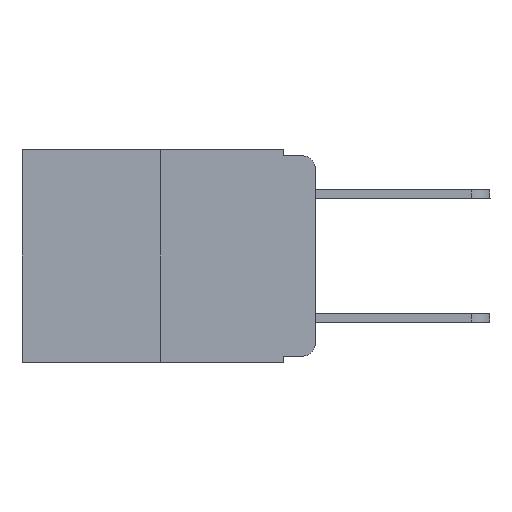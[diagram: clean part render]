
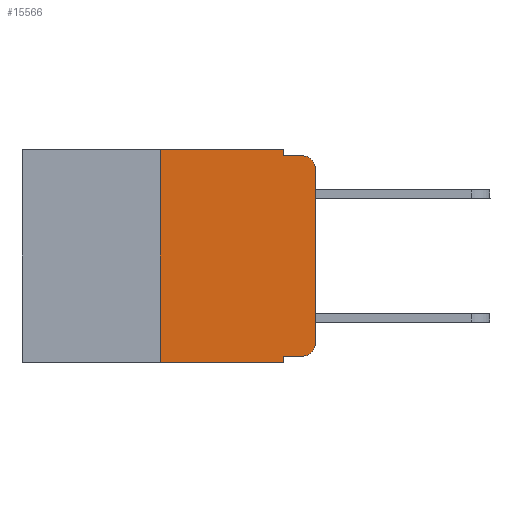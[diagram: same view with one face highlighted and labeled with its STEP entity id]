
A CAD part, left-side view. The second image highlights one B-rep face of the part: STEP entity #15566.
In plain terms, the highlighted planar face has unit normal (-1, 0, 0).
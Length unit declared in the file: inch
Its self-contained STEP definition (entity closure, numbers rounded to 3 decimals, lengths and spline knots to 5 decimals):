
#32 = DIRECTION ( 'NONE',  ( 0., -1., 0. ) ) ;
#188 = ORIENTED_EDGE ( 'NONE', *, *, #4467, .F. ) ;
#395 = LINE ( 'NONE', #13421, #13355 ) ;
#414 = CARTESIAN_POINT ( 'NONE',  ( 0., 0., -0.03 ) ) ;
#487 = EDGE_CURVE ( 'NONE', #4610, #6930, #16060, .T. ) ;
#597 = CIRCLE ( 'NONE', #18580, 0.02 ) ;
#861 = DIRECTION ( 'NONE',  ( -1., 0., 0. ) ) ;
#1271 = DIRECTION ( 'NONE',  ( 0., 0., -1. ) ) ;
#1429 = ORIENTED_EDGE ( 'NONE', *, *, #15662, .T. ) ;
#1655 = AXIS2_PLACEMENT_3D ( 'NONE', #23404, #861, #21895 ) ;
#1809 = VERTEX_POINT ( 'NONE', #8680 ) ;
#3310 = VECTOR ( 'NONE', #22823, 39.37008 ) ;
#3443 = EDGE_CURVE ( 'NONE', #19830, #23366, #395, .T. ) ;
#4153 = ORIENTED_EDGE ( 'NONE', *, *, #3443, .F. ) ;
#4163 = VECTOR ( 'NONE', #18431, 39.37008 ) ;
#4233 = CARTESIAN_POINT ( 'NONE',  ( 0., 0.02, -0.01 ) ) ;
#4467 = EDGE_CURVE ( 'NONE', #1809, #19830, #18538, .T. ) ;
#4527 = EDGE_CURVE ( 'NONE', #22119, #23366, #597, .T. ) ;
#4582 = CARTESIAN_POINT ( 'NONE',  ( 0., 0.473, 0. ) ) ;
#4610 = VERTEX_POINT ( 'NONE', #11165 ) ;
#4999 = EDGE_CURVE ( 'NONE', #16488, #4610, #7689, .T. ) ;
#5253 = DIRECTION ( 'NONE',  ( 0., -1., 0. ) ) ;
#5902 = EDGE_LOOP ( 'NONE', ( #6533, #13196, #4153, #188, #24316, #10038, #1429, #6755, #6245, #24729 ) ) ;
#6050 = VECTOR ( 'NONE', #5253, 39.37008 ) ;
#6245 = ORIENTED_EDGE ( 'NONE', *, *, #4999, .T. ) ;
#6533 = ORIENTED_EDGE ( 'NONE', *, *, #8102, .T. ) ;
#6610 = AXIS2_PLACEMENT_3D ( 'NONE', #4582, #23477, #23706 ) ;
#6755 = ORIENTED_EDGE ( 'NONE', *, *, #22675, .F. ) ;
#6930 = VERTEX_POINT ( 'NONE', #20135 ) ;
#6937 = DIRECTION ( 'NONE',  ( -1., 0., 0. ) ) ;
#7031 = CARTESIAN_POINT ( 'NONE',  ( 0., 0.051, 0. ) ) ;
#7160 = LINE ( 'NONE', #7031, #22132 ) ;
#7689 = LINE ( 'NONE', #7815, #20200 ) ;
#7815 = CARTESIAN_POINT ( 'NONE',  ( 0., 0.051, -0.333 ) ) ;
#8038 = DIRECTION ( 'NONE',  ( 0., -1., 0. ) ) ;
#8102 = EDGE_CURVE ( 'NONE', #6930, #22119, #17079, .T. ) ;
#8367 = VECTOR ( 'NONE', #24712, 39.37008 ) ;
#8680 = CARTESIAN_POINT ( 'NONE',  ( 0., 0.051, 0. ) ) ;
#8734 = CARTESIAN_POINT ( 'NONE',  ( 0., 0.051, -0.333 ) ) ;
#10038 = ORIENTED_EDGE ( 'NONE', *, *, #21927, .F. ) ;
#11165 = CARTESIAN_POINT ( 'NONE',  ( 0., 0.02, -0.333 ) ) ;
#11580 = CARTESIAN_POINT ( 'NONE',  ( 0., 0.051, -0.01 ) ) ;
#11805 = EDGE_CURVE ( 'NONE', #17230, #1809, #22141, .T. ) ;
#12421 = LINE ( 'NONE', #14210, #4163 ) ;
#12439 = VERTEX_POINT ( 'NONE', #13936 ) ;
#13035 = CARTESIAN_POINT ( 'NONE',  ( 0., 0.25, -0.343 ) ) ;
#13196 = ORIENTED_EDGE ( 'NONE', *, *, #4527, .T. ) ;
#13355 = VECTOR ( 'NONE', #8038, 39.37008 ) ;
#13421 = CARTESIAN_POINT ( 'NONE',  ( 0., 0.051, -0.01 ) ) ;
#13443 = CARTESIAN_POINT ( 'NONE',  ( 0., 0.25, 0. ) ) ;
#13936 = CARTESIAN_POINT ( 'NONE',  ( 0., 0.051, -0.343 ) ) ;
#14210 = CARTESIAN_POINT ( 'NONE',  ( 0., 0.473, -0.343 ) ) ;
#15566 = ADVANCED_FACE ( 'NONE', ( #21712 ), #21478, .F. ) ;
#15662 = EDGE_CURVE ( 'NONE', #17598, #12439, #12421, .T. ) ;
#16060 = CIRCLE ( 'NONE', #1655, 0.02 ) ;
#16488 = VERTEX_POINT ( 'NONE', #8734 ) ;
#17079 = LINE ( 'NONE', #18944, #8367 ) ;
#17230 = VERTEX_POINT ( 'NONE', #19437 ) ;
#17598 = VERTEX_POINT ( 'NONE', #13035 ) ;
#18431 = DIRECTION ( 'NONE',  ( 0., -1., 0. ) ) ;
#18538 = LINE ( 'NONE', #20051, #18973 ) ;
#18580 = AXIS2_PLACEMENT_3D ( 'NONE', #19941, #6937, #20307 ) ;
#18944 = CARTESIAN_POINT ( 'NONE',  ( 0., 0., 0. ) ) ;
#18973 = VECTOR ( 'NONE', #1271, 39.37008 ) ;
#19437 = CARTESIAN_POINT ( 'NONE',  ( 0., 0.25, 0. ) ) ;
#19830 = VERTEX_POINT ( 'NONE', #11580 ) ;
#19941 = CARTESIAN_POINT ( 'NONE',  ( 0., 0.02, -0.03 ) ) ;
#20051 = CARTESIAN_POINT ( 'NONE',  ( 0., 0.051, 0. ) ) ;
#20135 = CARTESIAN_POINT ( 'NONE',  ( 0., 0., -0.313 ) ) ;
#20200 = VECTOR ( 'NONE', #32, 39.37008 ) ;
#20265 = CARTESIAN_POINT ( 'NONE',  ( 0., 0.473, 0. ) ) ;
#20307 = DIRECTION ( 'NONE',  ( 0., 0., -1. ) ) ;
#20387 = DIRECTION ( 'NONE',  ( 0., 0., -1. ) ) ;
#21478 = PLANE ( 'NONE',  #6610 ) ;
#21712 = FACE_OUTER_BOUND ( 'NONE', #5902, .T. ) ;
#21895 = DIRECTION ( 'NONE',  ( 0., 0., -1. ) ) ;
#21927 = EDGE_CURVE ( 'NONE', #17598, #17230, #23081, .T. ) ;
#22119 = VERTEX_POINT ( 'NONE', #414 ) ;
#22132 = VECTOR ( 'NONE', #20387, 39.37008 ) ;
#22141 = LINE ( 'NONE', #20265, #6050 ) ;
#22675 = EDGE_CURVE ( 'NONE', #16488, #12439, #7160, .T. ) ;
#22823 = DIRECTION ( 'NONE',  ( 0., 0., 1. ) ) ;
#23081 = LINE ( 'NONE', #13443, #3310 ) ;
#23366 = VERTEX_POINT ( 'NONE', #4233 ) ;
#23404 = CARTESIAN_POINT ( 'NONE',  ( 0., 0.02, -0.313 ) ) ;
#23477 = DIRECTION ( 'NONE',  ( 1., 0., 0. ) ) ;
#23706 = DIRECTION ( 'NONE',  ( 0., 0., -1. ) ) ;
#24316 = ORIENTED_EDGE ( 'NONE', *, *, #11805, .F. ) ;
#24712 = DIRECTION ( 'NONE',  ( 0., 0., 1. ) ) ;
#24729 = ORIENTED_EDGE ( 'NONE', *, *, #487, .T. ) ;
